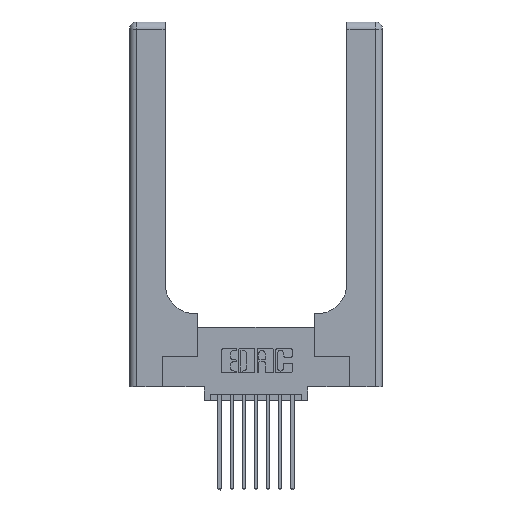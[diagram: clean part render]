
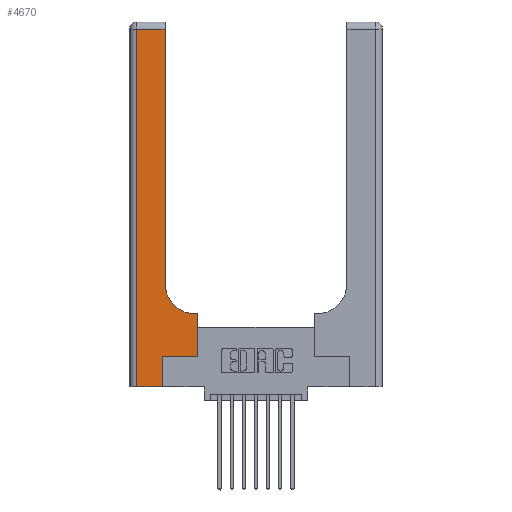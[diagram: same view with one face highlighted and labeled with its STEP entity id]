
A CAD part, top view. The second image highlights one B-rep face of the part: STEP entity #4670.
In plain terms, the highlighted planar face has unit normal (0, 0, 1).
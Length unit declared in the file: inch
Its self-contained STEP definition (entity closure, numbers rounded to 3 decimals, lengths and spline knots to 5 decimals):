
#22 = ORIENTED_EDGE ( 'NONE', *, *, #6842, .T. ) ;
#34 = FACE_OUTER_BOUND ( 'NONE', #5448, .T. ) ;
#88 = LINE ( 'NONE', #5486, #11571 ) ;
#525 = VERTEX_POINT ( 'NONE', #740 ) ;
#668 = VECTOR ( 'NONE', #873, 39.37008 ) ;
#681 = ORIENTED_EDGE ( 'NONE', *, *, #8622, .T. ) ;
#740 = CARTESIAN_POINT ( 'NONE',  ( 0.5585, 0.25, 0.37 ) ) ;
#873 = DIRECTION ( 'NONE',  ( 1., 0., 0. ) ) ;
#1242 = EDGE_CURVE ( 'NONE', #3779, #11025, #5238, .T. ) ;
#1361 = LINE ( 'NONE', #3418, #6032 ) ;
#1419 = ORIENTED_EDGE ( 'NONE', *, *, #7156, .T. ) ;
#1730 = EDGE_CURVE ( 'NONE', #9112, #10178, #2656, .T. ) ;
#1939 = CARTESIAN_POINT ( 'NONE',  ( 0.269, 0., 0.37 ) ) ;
#2188 = EDGE_CURVE ( 'NONE', #10178, #5362, #4963, .T. ) ;
#2369 = CARTESIAN_POINT ( 'NONE',  ( 0., 0., 0.37 ) ) ;
#2656 = LINE ( 'NONE', #2369, #5429 ) ;
#2939 = LINE ( 'NONE', #13951, #668 ) ;
#2952 = ORIENTED_EDGE ( 'NONE', *, *, #14511, .T. ) ;
#2989 = CARTESIAN_POINT ( 'NONE',  ( 0.2915, 0.85, 0.37 ) ) ;
#3418 = CARTESIAN_POINT ( 'NONE',  ( 0.06, 3., 0.37 ) ) ;
#3779 = VERTEX_POINT ( 'NONE', #10325 ) ;
#4281 = DIRECTION ( 'NONE',  ( 0., 1., 0. ) ) ;
#4401 = CARTESIAN_POINT ( 'NONE',  ( 0.06, 2.94, 0.37 ) ) ;
#4406 = PLANE ( 'NONE',  #5383 ) ;
#4522 = EDGE_CURVE ( 'NONE', #15198, #9112, #1361, .T. ) ;
#4620 = DIRECTION ( 'NONE',  ( 0., 0., -1. ) ) ;
#4670 = ADVANCED_FACE ( 'NONE', ( #34 ), #4406, .F. ) ;
#4963 = LINE ( 'NONE', #8976, #5713 ) ;
#5238 = CIRCLE ( 'NONE', #6760, 0.25 ) ;
#5337 = LINE ( 'NONE', #9304, #7793 ) ;
#5362 = VERTEX_POINT ( 'NONE', #12024 ) ;
#5383 = AXIS2_PLACEMENT_3D ( 'NONE', #10609, #4620, #9264 ) ;
#5429 = VECTOR ( 'NONE', #11803, 39.37008 ) ;
#5448 = EDGE_LOOP ( 'NONE', ( #681, #2952, #15223, #15307, #9365, #14501, #1419, #22, #11788 ) ) ;
#5486 = CARTESIAN_POINT ( 'NONE',  ( 0., 2.94, 0.37 ) ) ;
#5571 = DIRECTION ( 'NONE',  ( 0., 1., 0. ) ) ;
#5643 = CARTESIAN_POINT ( 'NONE',  ( 0.2915, 2.94, 0.37 ) ) ;
#5713 = VECTOR ( 'NONE', #4281, 39.37008 ) ;
#6032 = VECTOR ( 'NONE', #15286, 39.37008 ) ;
#6145 = LINE ( 'NONE', #12008, #13138 ) ;
#6760 = AXIS2_PLACEMENT_3D ( 'NONE', #8170, #10612, #9418 ) ;
#6842 = EDGE_CURVE ( 'NONE', #12038, #3779, #6145, .T. ) ;
#7014 = CARTESIAN_POINT ( 'NONE',  ( 0.5585, 0.6, 0.37 ) ) ;
#7156 = EDGE_CURVE ( 'NONE', #525, #12038, #11825, .T. ) ;
#7793 = VECTOR ( 'NONE', #5571, 39.37008 ) ;
#8170 = CARTESIAN_POINT ( 'NONE',  ( 0.5415, 0.85, 0.37 ) ) ;
#8224 = DIRECTION ( 'NONE',  ( 0., 1., 0. ) ) ;
#8581 = VECTOR ( 'NONE', #8224, 39.37008 ) ;
#8622 = EDGE_CURVE ( 'NONE', #11025, #13748, #5337, .T. ) ;
#8647 = EDGE_CURVE ( 'NONE', #5362, #525, #2939, .T. ) ;
#8901 = DIRECTION ( 'NONE',  ( -1., 0., 0. ) ) ;
#8976 = CARTESIAN_POINT ( 'NONE',  ( 0.269, 0., 0.37 ) ) ;
#9112 = VERTEX_POINT ( 'NONE', #12332 ) ;
#9264 = DIRECTION ( 'NONE',  ( -1., 0., 0. ) ) ;
#9304 = CARTESIAN_POINT ( 'NONE',  ( 0.2915, 3., 0.37 ) ) ;
#9365 = ORIENTED_EDGE ( 'NONE', *, *, #2188, .T. ) ;
#9418 = DIRECTION ( 'NONE',  ( 1., 0., 0. ) ) ;
#10178 = VERTEX_POINT ( 'NONE', #1939 ) ;
#10325 = CARTESIAN_POINT ( 'NONE',  ( 0.5415, 0.6, 0.37 ) ) ;
#10609 = CARTESIAN_POINT ( 'NONE',  ( 0., 3., 0.37 ) ) ;
#10612 = DIRECTION ( 'NONE',  ( 0., 0., -1. ) ) ;
#10721 = CARTESIAN_POINT ( 'NONE',  ( 0.5585, 0.25, 0.37 ) ) ;
#10752 = DIRECTION ( 'NONE',  ( -1., 0., 0. ) ) ;
#11025 = VERTEX_POINT ( 'NONE', #2989 ) ;
#11571 = VECTOR ( 'NONE', #8901, 39.37008 ) ;
#11788 = ORIENTED_EDGE ( 'NONE', *, *, #1242, .T. ) ;
#11803 = DIRECTION ( 'NONE',  ( 1., 0., 0. ) ) ;
#11825 = LINE ( 'NONE', #10721, #8581 ) ;
#12008 = CARTESIAN_POINT ( 'NONE',  ( 0.2915, 0.6, 0.37 ) ) ;
#12024 = CARTESIAN_POINT ( 'NONE',  ( 0.269, 0.25, 0.37 ) ) ;
#12038 = VERTEX_POINT ( 'NONE', #7014 ) ;
#12332 = CARTESIAN_POINT ( 'NONE',  ( 0.06, 0., 0.37 ) ) ;
#13138 = VECTOR ( 'NONE', #10752, 39.37008 ) ;
#13748 = VERTEX_POINT ( 'NONE', #5643 ) ;
#13951 = CARTESIAN_POINT ( 'NONE',  ( 0.269, 0.25, 0.37 ) ) ;
#14501 = ORIENTED_EDGE ( 'NONE', *, *, #8647, .T. ) ;
#14511 = EDGE_CURVE ( 'NONE', #13748, #15198, #88, .T. ) ;
#15198 = VERTEX_POINT ( 'NONE', #4401 ) ;
#15223 = ORIENTED_EDGE ( 'NONE', *, *, #4522, .T. ) ;
#15286 = DIRECTION ( 'NONE',  ( 0., -1., 0. ) ) ;
#15307 = ORIENTED_EDGE ( 'NONE', *, *, #1730, .T. ) ;
